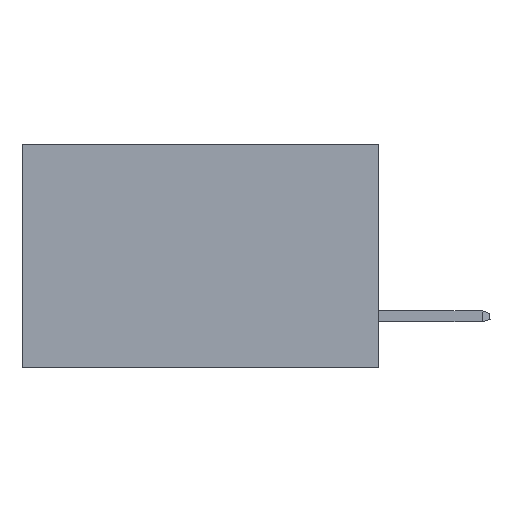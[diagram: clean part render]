
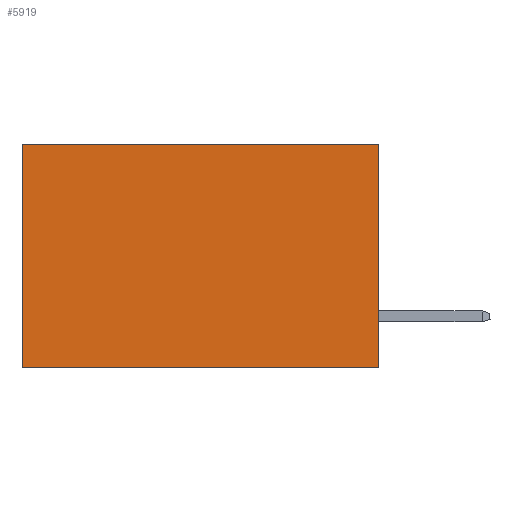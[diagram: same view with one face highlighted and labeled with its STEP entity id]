
A CAD part, left-side view. The second image highlights one B-rep face of the part: STEP entity #5919.
In plain terms, the highlighted planar face has unit normal (-1, 0, 0).
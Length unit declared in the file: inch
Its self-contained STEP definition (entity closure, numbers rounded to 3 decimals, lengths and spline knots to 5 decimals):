
#1152 = AXIS2_PLACEMENT_3D ( 'NONE', #16983, #16563, #16545 ) ;
#2494 = LINE ( 'NONE', #10022, #6696 ) ;
#2688 = EDGE_CURVE ( 'NONE', #17123, #9559, #7564, .T. ) ;
#2983 = CARTESIAN_POINT ( 'NONE',  ( 0.277, 0.59, -0.37 ) ) ;
#3325 = CARTESIAN_POINT ( 'NONE',  ( 0.277, 0.59, -0.37 ) ) ;
#3333 = VECTOR ( 'NONE', #3921, 39.37008 ) ;
#3652 = DIRECTION ( 'NONE',  ( 0., 0., -1. ) ) ;
#3921 = DIRECTION ( 'NONE',  ( 0., 1., 0. ) ) ;
#4020 = VERTEX_POINT ( 'NONE', #2983 ) ;
#5836 = CARTESIAN_POINT ( 'NONE',  ( 0.277, 0.59, 0. ) ) ;
#5919 = ADVANCED_FACE ( 'NONE', ( #5981 ), #16873, .F. ) ;
#5981 = FACE_OUTER_BOUND ( 'NONE', #6600, .T. ) ;
#6411 = VECTOR ( 'NONE', #3652, 39.37008 ) ;
#6509 = EDGE_CURVE ( 'NONE', #17123, #20361, #19368, .T. ) ;
#6600 = EDGE_LOOP ( 'NONE', ( #11972, #14935, #11994, #16197 ) ) ;
#6673 = VECTOR ( 'NONE', #10326, 39.37008 ) ;
#6696 = VECTOR ( 'NONE', #13158, 39.37008 ) ;
#7141 = EDGE_CURVE ( 'NONE', #9559, #4020, #7402, .T. ) ;
#7402 = LINE ( 'NONE', #3325, #6411 ) ;
#7564 = LINE ( 'NONE', #9707, #3333 ) ;
#8085 = CARTESIAN_POINT ( 'NONE',  ( 0.277, 0., -0.37 ) ) ;
#9559 = VERTEX_POINT ( 'NONE', #5836 ) ;
#9707 = CARTESIAN_POINT ( 'NONE',  ( 0.277, 0., 0. ) ) ;
#10022 = CARTESIAN_POINT ( 'NONE',  ( 0.277, 0., -0.37 ) ) ;
#10326 = DIRECTION ( 'NONE',  ( 0., 0., -1. ) ) ;
#10438 = CARTESIAN_POINT ( 'NONE',  ( 0.277, 0., -0.37 ) ) ;
#11972 = ORIENTED_EDGE ( 'NONE', *, *, #7141, .T. ) ;
#11994 = ORIENTED_EDGE ( 'NONE', *, *, #6509, .F. ) ;
#13158 = DIRECTION ( 'NONE',  ( 0., 1., 0. ) ) ;
#13364 = CARTESIAN_POINT ( 'NONE',  ( 0.277, 0., 0. ) ) ;
#14935 = ORIENTED_EDGE ( 'NONE', *, *, #17057, .F. ) ;
#16197 = ORIENTED_EDGE ( 'NONE', *, *, #2688, .T. ) ;
#16545 = DIRECTION ( 'NONE',  ( 0., 0., -1. ) ) ;
#16563 = DIRECTION ( 'NONE',  ( 1., 0., 0. ) ) ;
#16873 = PLANE ( 'NONE',  #1152 ) ;
#16983 = CARTESIAN_POINT ( 'NONE',  ( 0.277, 0., -0.37 ) ) ;
#17057 = EDGE_CURVE ( 'NONE', #20361, #4020, #2494, .T. ) ;
#17123 = VERTEX_POINT ( 'NONE', #13364 ) ;
#19368 = LINE ( 'NONE', #10438, #6673 ) ;
#20361 = VERTEX_POINT ( 'NONE', #8085 ) ;
